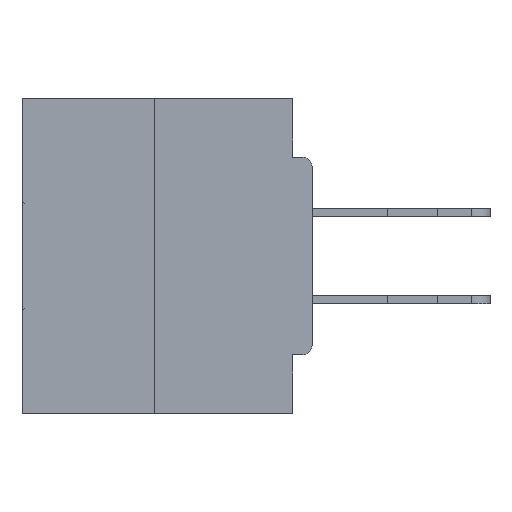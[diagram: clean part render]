
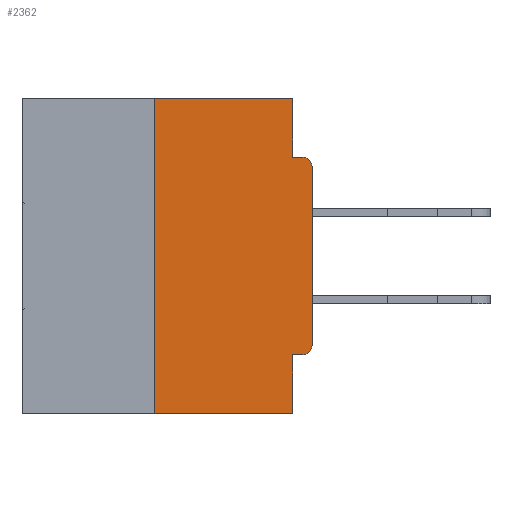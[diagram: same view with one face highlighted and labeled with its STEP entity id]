
A CAD part, left-side view. The second image highlights one B-rep face of the part: STEP entity #2362.
In plain terms, the highlighted planar face has unit normal (-1, 0, 0).
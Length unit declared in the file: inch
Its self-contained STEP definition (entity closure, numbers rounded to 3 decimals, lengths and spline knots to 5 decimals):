
#614 = LINE ( 'NONE', #32828, #28584 ) ;
#954 = DIRECTION ( 'NONE',  ( 1., 0., 0. ) ) ;
#1123 = EDGE_CURVE ( 'NONE', #41336, #29158, #2227, .T. ) ;
#1910 = CARTESIAN_POINT ( 'NONE',  ( 0., 0.031, -0.0935 ) ) ;
#2173 = LINE ( 'NONE', #23916, #33615 ) ;
#2227 = LINE ( 'NONE', #3794, #18992 ) ;
#2362 = ADVANCED_FACE ( 'NONE', ( #27542 ), #24139, .F. ) ;
#3518 = ORIENTED_EDGE ( 'NONE', *, *, #26713, .T. ) ;
#3566 = EDGE_CURVE ( 'NONE', #9632, #29158, #32418, .T. ) ;
#3794 = CARTESIAN_POINT ( 'NONE',  ( 0., 0.031, -0.5 ) ) ;
#4238 = EDGE_CURVE ( 'NONE', #9199, #39549, #11095, .T. ) ;
#4826 = DIRECTION ( 'NONE',  ( 0., 0., -1. ) ) ;
#5038 = DIRECTION ( 'NONE',  ( 0., -1., 0. ) ) ;
#5879 = CARTESIAN_POINT ( 'NONE',  ( 0., 0.031, -0.4065 ) ) ;
#6442 = CARTESIAN_POINT ( 'NONE',  ( 0., 0.015, -0.4065 ) ) ;
#6461 = LINE ( 'NONE', #32856, #36902 ) ;
#7805 = LINE ( 'NONE', #30179, #28611 ) ;
#8128 = ORIENTED_EDGE ( 'NONE', *, *, #3566, .T. ) ;
#8539 = VECTOR ( 'NONE', #42057, 39.37008 ) ;
#9199 = VERTEX_POINT ( 'NONE', #12516 ) ;
#9610 = DIRECTION ( 'NONE',  ( 0., -1., 0. ) ) ;
#9632 = VERTEX_POINT ( 'NONE', #18407 ) ;
#10040 = DIRECTION ( 'NONE',  ( 0., 0., -1. ) ) ;
#11065 = DIRECTION ( 'NONE',  ( 0., 1., 0. ) ) ;
#11095 = CIRCLE ( 'NONE', #36608, 0.015 ) ;
#11277 = CARTESIAN_POINT ( 'NONE',  ( 0., 0.46, -0.5 ) ) ;
#12366 = VERTEX_POINT ( 'NONE', #22088 ) ;
#12516 = CARTESIAN_POINT ( 'NONE',  ( 0., 0., -0.1085 ) ) ;
#13997 = DIRECTION ( 'NONE',  ( 0., -1., 0. ) ) ;
#16148 = ORIENTED_EDGE ( 'NONE', *, *, #17918, .F. ) ;
#16222 = VERTEX_POINT ( 'NONE', #6442 ) ;
#17323 = EDGE_CURVE ( 'NONE', #9632, #24868, #7805, .T. ) ;
#17452 = CIRCLE ( 'NONE', #41140, 0.015 ) ;
#17918 = EDGE_CURVE ( 'NONE', #21979, #39549, #2173, .T. ) ;
#18218 = EDGE_CURVE ( 'NONE', #12366, #9199, #24482, .T. ) ;
#18407 = CARTESIAN_POINT ( 'NONE',  ( 0., 0.25, -0.5 ) ) ;
#18990 = EDGE_CURVE ( 'NONE', #41019, #21979, #34382, .T. ) ;
#18992 = VECTOR ( 'NONE', #10040, 39.37008 ) ;
#20400 = VECTOR ( 'NONE', #34675, 39.37008 ) ;
#20853 = ORIENTED_EDGE ( 'NONE', *, *, #18218, .T. ) ;
#21415 = CARTESIAN_POINT ( 'NONE',  ( 0., 0.015, -0.1085 ) ) ;
#21812 = ORIENTED_EDGE ( 'NONE', *, *, #18990, .F. ) ;
#21951 = ORIENTED_EDGE ( 'NONE', *, *, #40591, .F. ) ;
#21979 = VERTEX_POINT ( 'NONE', #1910 ) ;
#22088 = CARTESIAN_POINT ( 'NONE',  ( 0., 0., -0.3915 ) ) ;
#23059 = ORIENTED_EDGE ( 'NONE', *, *, #1123, .F. ) ;
#23781 = DIRECTION ( 'NONE',  ( 0., 0., 1. ) ) ;
#23916 = CARTESIAN_POINT ( 'NONE',  ( 0., 0., -0.0935 ) ) ;
#24137 = ORIENTED_EDGE ( 'NONE', *, *, #4238, .T. ) ;
#24139 = PLANE ( 'NONE',  #35721 ) ;
#24482 = LINE ( 'NONE', #31711, #20400 ) ;
#24868 = VERTEX_POINT ( 'NONE', #33135 ) ;
#25450 = CARTESIAN_POINT ( 'NONE',  ( 0., 0.031, 0. ) ) ;
#25454 = EDGE_CURVE ( 'NONE', #16222, #41336, #6461, .T. ) ;
#25853 = ORIENTED_EDGE ( 'NONE', *, *, #25454, .F. ) ;
#26713 = EDGE_CURVE ( 'NONE', #16222, #12366, #17452, .T. ) ;
#27181 = DIRECTION ( 'NONE',  ( -1., 0., 0. ) ) ;
#27542 = FACE_OUTER_BOUND ( 'NONE', #31128, .T. ) ;
#28584 = VECTOR ( 'NONE', #9610, 39.37008 ) ;
#28611 = VECTOR ( 'NONE', #23781, 39.37008 ) ;
#29158 = VERTEX_POINT ( 'NONE', #37479 ) ;
#30179 = CARTESIAN_POINT ( 'NONE',  ( 0., 0.25, 0. ) ) ;
#30806 = DIRECTION ( 'NONE',  ( 0., 0., -1. ) ) ;
#31128 = EDGE_LOOP ( 'NONE', ( #21951, #40174, #8128, #23059, #25853, #3518, #20853, #24137, #16148, #21812 ) ) ;
#31711 = CARTESIAN_POINT ( 'NONE',  ( 0., 0., 0. ) ) ;
#32418 = LINE ( 'NONE', #11277, #37556 ) ;
#32828 = CARTESIAN_POINT ( 'NONE',  ( 0., 0.46, 0. ) ) ;
#32856 = CARTESIAN_POINT ( 'NONE',  ( 0., 0., -0.4065 ) ) ;
#33135 = CARTESIAN_POINT ( 'NONE',  ( 0., 0.25, 0. ) ) ;
#33615 = VECTOR ( 'NONE', #13997, 39.37008 ) ;
#33667 = DIRECTION ( 'NONE',  ( 0., 0., -1. ) ) ;
#34163 = DIRECTION ( 'NONE',  ( -1., 0., 0. ) ) ;
#34382 = LINE ( 'NONE', #38523, #8539 ) ;
#34675 = DIRECTION ( 'NONE',  ( 0., 0., 1. ) ) ;
#35721 = AXIS2_PLACEMENT_3D ( 'NONE', #37219, #954, #4826 ) ;
#36608 = AXIS2_PLACEMENT_3D ( 'NONE', #21415, #34163, #30806 ) ;
#36902 = VECTOR ( 'NONE', #11065, 39.37008 ) ;
#37219 = CARTESIAN_POINT ( 'NONE',  ( 0., 0.46, 0. ) ) ;
#37479 = CARTESIAN_POINT ( 'NONE',  ( 0., 0.031, -0.5 ) ) ;
#37556 = VECTOR ( 'NONE', #5038, 39.37008 ) ;
#38523 = CARTESIAN_POINT ( 'NONE',  ( 0., 0.031, 0. ) ) ;
#39549 = VERTEX_POINT ( 'NONE', #41731 ) ;
#40174 = ORIENTED_EDGE ( 'NONE', *, *, #17323, .F. ) ;
#40358 = CARTESIAN_POINT ( 'NONE',  ( 0., 0.015, -0.3915 ) ) ;
#40591 = EDGE_CURVE ( 'NONE', #24868, #41019, #614, .T. ) ;
#41019 = VERTEX_POINT ( 'NONE', #25450 ) ;
#41140 = AXIS2_PLACEMENT_3D ( 'NONE', #40358, #27181, #33667 ) ;
#41336 = VERTEX_POINT ( 'NONE', #5879 ) ;
#41731 = CARTESIAN_POINT ( 'NONE',  ( 0., 0.015, -0.0935 ) ) ;
#42057 = DIRECTION ( 'NONE',  ( 0., 0., -1. ) ) ;
